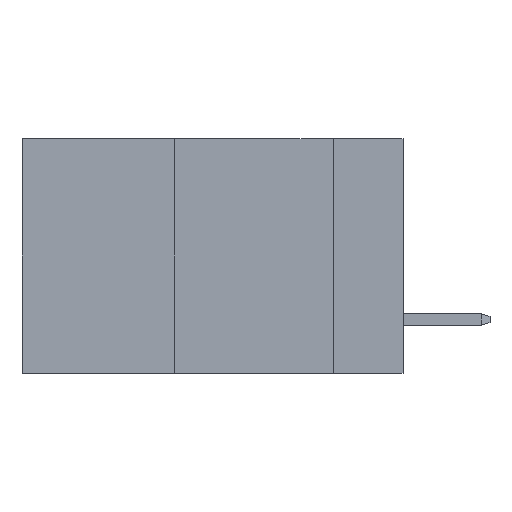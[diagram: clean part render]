
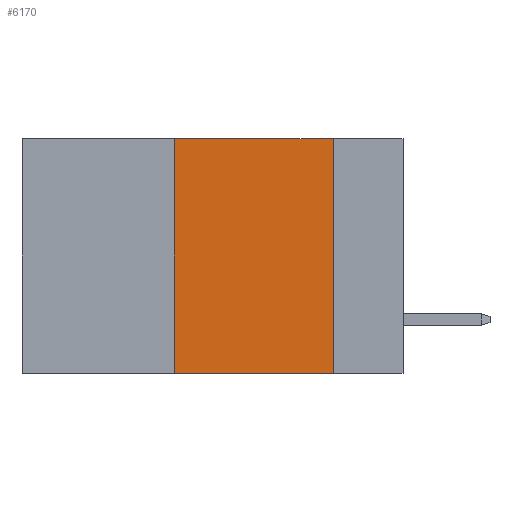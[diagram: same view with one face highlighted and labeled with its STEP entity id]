
A CAD part, left-side view. The second image highlights one B-rep face of the part: STEP entity #6170.
In plain terms, the highlighted planar face has unit normal (-1, 0, 0).
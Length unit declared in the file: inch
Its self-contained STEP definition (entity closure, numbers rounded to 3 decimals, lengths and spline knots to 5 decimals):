
#164 = VERTEX_POINT ( 'NONE', #6205 ) ;
#369 = CARTESIAN_POINT ( 'NONE',  ( 0., 0.6, -0.37 ) ) ;
#784 = DIRECTION ( 'NONE',  ( 0., 0., -1. ) ) ;
#1857 = CARTESIAN_POINT ( 'NONE',  ( 0., 0.11, 0. ) ) ;
#2187 = AXIS2_PLACEMENT_3D ( 'NONE', #11071, #7569, #8941 ) ;
#2557 = VERTEX_POINT ( 'NONE', #12651 ) ;
#2649 = ORIENTED_EDGE ( 'NONE', *, *, #11945, .F. ) ;
#2670 = ORIENTED_EDGE ( 'NONE', *, *, #10510, .F. ) ;
#3654 = CARTESIAN_POINT ( 'NONE',  ( 0., 0.6, 0. ) ) ;
#3717 = ORIENTED_EDGE ( 'NONE', *, *, #6707, .F. ) ;
#4389 = LINE ( 'NONE', #4464, #6939 ) ;
#4391 = CARTESIAN_POINT ( 'NONE',  ( 0., 0.11, -0.37 ) ) ;
#4464 = CARTESIAN_POINT ( 'NONE',  ( 0., 0.36, 0. ) ) ;
#5227 = EDGE_CURVE ( 'NONE', #164, #11023, #5864, .T. ) ;
#5864 = LINE ( 'NONE', #369, #6195 ) ;
#6170 = ADVANCED_FACE ( 'NONE', ( #12293 ), #12206, .F. ) ;
#6195 = VECTOR ( 'NONE', #7021, 39.37008 ) ;
#6205 = CARTESIAN_POINT ( 'NONE',  ( 0., 0.36, -0.37 ) ) ;
#6707 = EDGE_CURVE ( 'NONE', #13405, #11023, #12392, .T. ) ;
#6939 = VECTOR ( 'NONE', #9134, 39.37008 ) ;
#7021 = DIRECTION ( 'NONE',  ( 0., -1., 0. ) ) ;
#7569 = DIRECTION ( 'NONE',  ( 1., 0., 0. ) ) ;
#8941 = DIRECTION ( 'NONE',  ( 0., 0., -1. ) ) ;
#9134 = DIRECTION ( 'NONE',  ( 0., 0., 1. ) ) ;
#10510 = EDGE_CURVE ( 'NONE', #164, #2557, #4389, .T. ) ;
#11023 = VERTEX_POINT ( 'NONE', #4391 ) ;
#11071 = CARTESIAN_POINT ( 'NONE',  ( 0., 0.6, 0. ) ) ;
#11945 = EDGE_CURVE ( 'NONE', #2557, #13405, #12836, .T. ) ;
#12200 = CARTESIAN_POINT ( 'NONE',  ( 0., 0.11, 0. ) ) ;
#12206 = PLANE ( 'NONE',  #2187 ) ;
#12293 = FACE_OUTER_BOUND ( 'NONE', #12349, .T. ) ;
#12349 = EDGE_LOOP ( 'NONE', ( #3717, #2649, #2670, #13099 ) ) ;
#12392 = LINE ( 'NONE', #1857, #14162 ) ;
#12651 = CARTESIAN_POINT ( 'NONE',  ( 0., 0.36, 0. ) ) ;
#12676 = DIRECTION ( 'NONE',  ( 0., -1., 0. ) ) ;
#12836 = LINE ( 'NONE', #3654, #14990 ) ;
#13099 = ORIENTED_EDGE ( 'NONE', *, *, #5227, .T. ) ;
#13405 = VERTEX_POINT ( 'NONE', #12200 ) ;
#14162 = VECTOR ( 'NONE', #784, 39.37008 ) ;
#14990 = VECTOR ( 'NONE', #12676, 39.37008 ) ;
